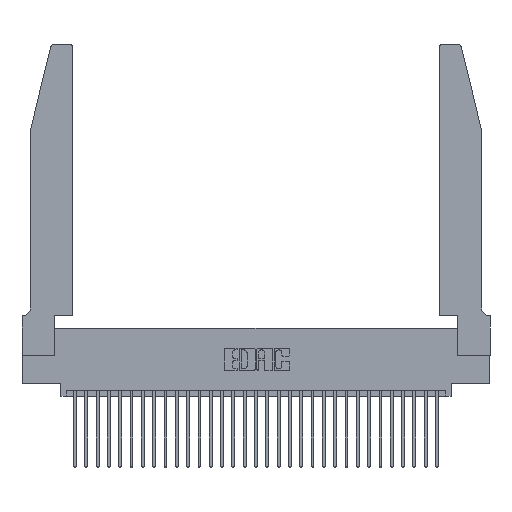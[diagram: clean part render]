
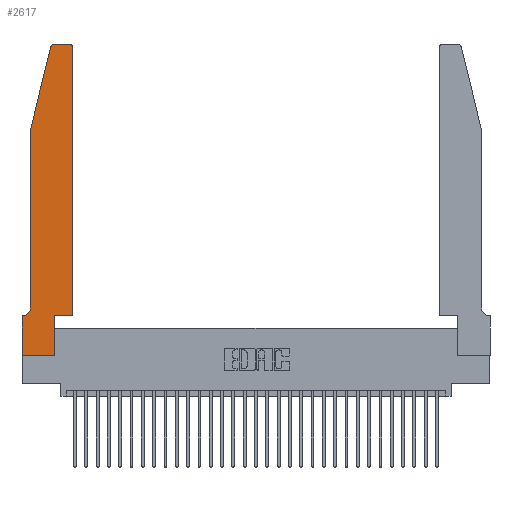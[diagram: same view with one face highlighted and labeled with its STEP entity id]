
A CAD part, top view. The second image highlights one B-rep face of the part: STEP entity #2617.
In plain terms, the highlighted planar face has unit normal (0, 0, 1).
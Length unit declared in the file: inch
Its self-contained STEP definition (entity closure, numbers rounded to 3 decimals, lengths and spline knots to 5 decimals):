
#108 = ORIENTED_EDGE ( 'NONE', *, *, #10033, .T. ) ;
#432 = EDGE_CURVE ( 'NONE', #23651, #25471, #24129, .T. ) ;
#804 = DIRECTION ( 'NONE',  ( 1., 0., 0. ) ) ;
#1020 = CARTESIAN_POINT ( 'NONE',  ( 0., 0., 0.37 ) ) ;
#1551 = DIRECTION ( 'NONE',  ( -1., 0., 0. ) ) ;
#2395 = DIRECTION ( 'NONE',  ( 0., 0., 1. ) ) ;
#2446 = CARTESIAN_POINT ( 'NONE',  ( 0., 0., 0.37 ) ) ;
#2617 = ADVANCED_FACE ( 'NONE', ( #11401 ), #15504, .T. ) ;
#2775 = VECTOR ( 'NONE', #18620, 39.37008 ) ;
#3001 = EDGE_CURVE ( 'NONE', #5700, #26928, #12154, .T. ) ;
#3244 = DIRECTION ( 'NONE',  ( 0., 0., 1. ) ) ;
#3672 = EDGE_LOOP ( 'NONE', ( #5159, #108, #13438, #28857, #13011, #16628, #20167, #29893, #7004, #9780, #23713, #18975 ) ) ;
#4205 = AXIS2_PLACEMENT_3D ( 'NONE', #13001, #25788, #13106 ) ;
#4511 = DIRECTION ( 'NONE',  ( 0., 1., 0. ) ) ;
#4675 = EDGE_CURVE ( 'NONE', #8974, #28708, #5475, .T. ) ;
#4848 = VECTOR ( 'NONE', #4511, 39.37008 ) ;
#5159 = ORIENTED_EDGE ( 'NONE', *, *, #432, .T. ) ;
#5475 = LINE ( 'NONE', #11590, #22478 ) ;
#5673 = CARTESIAN_POINT ( 'NONE',  ( 0.284, 2.75, 0.37 ) ) ;
#5700 = VERTEX_POINT ( 'NONE', #26299 ) ;
#6003 = EDGE_CURVE ( 'NONE', #9294, #23651, #8084, .T. ) ;
#6715 = CARTESIAN_POINT ( 'NONE',  ( 0.0755, 2., 0.37 ) ) ;
#7004 = ORIENTED_EDGE ( 'NONE', *, *, #14526, .T. ) ;
#7499 = VECTOR ( 'NONE', #25709, 39.37008 ) ;
#7746 = VERTEX_POINT ( 'NONE', #14451 ) ;
#7762 = VECTOR ( 'NONE', #28252, 39.37008 ) ;
#8084 = CIRCLE ( 'NONE', #23474, 0.03 ) ;
#8286 = CARTESIAN_POINT ( 'NONE',  ( 0.4205, 2.72, 0.37 ) ) ;
#8386 = CARTESIAN_POINT ( 'NONE',  ( 0.4505, 0.35, 0.37 ) ) ;
#8974 = VERTEX_POINT ( 'NONE', #6715 ) ;
#9065 = CARTESIAN_POINT ( 'NONE',  ( 0.0755, 0.35, 0.37 ) ) ;
#9294 = VERTEX_POINT ( 'NONE', #9440 ) ;
#9440 = CARTESIAN_POINT ( 'NONE',  ( 0.4505, 2.72, 0.37 ) ) ;
#9780 = ORIENTED_EDGE ( 'NONE', *, *, #18970, .T. ) ;
#10033 = EDGE_CURVE ( 'NONE', #25471, #27442, #21724, .T. ) ;
#11401 = FACE_OUTER_BOUND ( 'NONE', #3672, .T. ) ;
#11590 = CARTESIAN_POINT ( 'NONE',  ( 0.0755, 2., 0.37 ) ) ;
#12142 = DIRECTION ( 'NONE',  ( 0., -1., 0. ) ) ;
#12154 = LINE ( 'NONE', #2446, #27236 ) ;
#12492 = DIRECTION ( 'NONE',  ( 0., 0., -1. ) ) ;
#12858 = VERTEX_POINT ( 'NONE', #18215 ) ;
#13001 = CARTESIAN_POINT ( 'NONE',  ( 0., 0.35, 0.37 ) ) ;
#13011 = ORIENTED_EDGE ( 'NONE', *, *, #18200, .T. ) ;
#13106 = DIRECTION ( 'NONE',  ( 1., 0., 0. ) ) ;
#13399 = VECTOR ( 'NONE', #804, 39.37008 ) ;
#13438 = ORIENTED_EDGE ( 'NONE', *, *, #19092, .T. ) ;
#13456 = EDGE_CURVE ( 'NONE', #26928, #12858, #19979, .T. ) ;
#14301 = VECTOR ( 'NONE', #26373, 39.37008 ) ;
#14451 = CARTESIAN_POINT ( 'NONE',  ( 0.2865, 0.35, 0.37 ) ) ;
#14526 = EDGE_CURVE ( 'NONE', #12858, #7746, #31569, .T. ) ;
#14650 = DIRECTION ( 'NONE',  ( -1., 0., 0. ) ) ;
#15427 = CARTESIAN_POINT ( 'NONE',  ( 0.25487, 2.72718, 0.37 ) ) ;
#15504 = PLANE ( 'NONE',  #4205 ) ;
#16032 = VERTEX_POINT ( 'NONE', #28090 ) ;
#16333 = CIRCLE ( 'NONE', #31614, 0.07 ) ;
#16628 = ORIENTED_EDGE ( 'NONE', *, *, #19931, .T. ) ;
#16662 = LINE ( 'NONE', #18415, #7762 ) ;
#17142 = CARTESIAN_POINT ( 'NONE',  ( 0.0055, 0.42, 0.37 ) ) ;
#17158 = CARTESIAN_POINT ( 'NONE',  ( 0.284, 2.72, 0.37 ) ) ;
#17810 = DIRECTION ( 'NONE',  ( 1., 0., 0. ) ) ;
#18200 = EDGE_CURVE ( 'NONE', #28708, #16032, #16333, .T. ) ;
#18215 = CARTESIAN_POINT ( 'NONE',  ( 0.2865, 0., 0.37 ) ) ;
#18336 = LINE ( 'NONE', #8386, #7499 ) ;
#18415 = CARTESIAN_POINT ( 'NONE',  ( 0.4505, 0.35, 0.37 ) ) ;
#18620 = DIRECTION ( 'NONE',  ( -0.239, -0.971, 0. ) ) ;
#18970 = EDGE_CURVE ( 'NONE', #7746, #19333, #16662, .T. ) ;
#18975 = ORIENTED_EDGE ( 'NONE', *, *, #6003, .T. ) ;
#19041 = CARTESIAN_POINT ( 'NONE',  ( 0.2605, 2.75, 0.37 ) ) ;
#19092 = EDGE_CURVE ( 'NONE', #27442, #8974, #22066, .T. ) ;
#19333 = VERTEX_POINT ( 'NONE', #29322 ) ;
#19476 = DIRECTION ( 'NONE',  ( 0., -1., 0. ) ) ;
#19931 = EDGE_CURVE ( 'NONE', #16032, #5700, #31381, .T. ) ;
#19979 = LINE ( 'NONE', #1020, #13399 ) ;
#20167 = ORIENTED_EDGE ( 'NONE', *, *, #3001, .T. ) ;
#20431 = AXIS2_PLACEMENT_3D ( 'NONE', #17158, #2395, #25366 ) ;
#21307 = CARTESIAN_POINT ( 'NONE',  ( 0.0755, 2., 0.37 ) ) ;
#21724 = CIRCLE ( 'NONE', #20431, 0.03 ) ;
#21886 = CARTESIAN_POINT ( 'NONE',  ( 0.2865, 0.35, 0.37 ) ) ;
#22066 = LINE ( 'NONE', #21307, #2775 ) ;
#22478 = VECTOR ( 'NONE', #19476, 39.37008 ) ;
#23474 = AXIS2_PLACEMENT_3D ( 'NONE', #8286, #3244, #17810 ) ;
#23651 = VERTEX_POINT ( 'NONE', #25107 ) ;
#23713 = ORIENTED_EDGE ( 'NONE', *, *, #26663, .T. ) ;
#24129 = LINE ( 'NONE', #19041, #29970 ) ;
#25107 = CARTESIAN_POINT ( 'NONE',  ( 0.4205, 2.75, 0.37 ) ) ;
#25366 = DIRECTION ( 'NONE',  ( 1., 0., 0. ) ) ;
#25471 = VERTEX_POINT ( 'NONE', #5673 ) ;
#25651 = CARTESIAN_POINT ( 'NONE',  ( 0.0755, 0.42, 0.37 ) ) ;
#25709 = DIRECTION ( 'NONE',  ( 0., 1., 0. ) ) ;
#25788 = DIRECTION ( 'NONE',  ( 0., 0., 1. ) ) ;
#26299 = CARTESIAN_POINT ( 'NONE',  ( 0., 0.35, 0.37 ) ) ;
#26373 = DIRECTION ( 'NONE',  ( -1., 0., 0. ) ) ;
#26663 = EDGE_CURVE ( 'NONE', #19333, #9294, #18336, .T. ) ;
#26884 = CARTESIAN_POINT ( 'NONE',  ( 0., 0., 0.37 ) ) ;
#26928 = VERTEX_POINT ( 'NONE', #26884 ) ;
#27236 = VECTOR ( 'NONE', #12142, 39.37008 ) ;
#27442 = VERTEX_POINT ( 'NONE', #15427 ) ;
#28090 = CARTESIAN_POINT ( 'NONE',  ( 0.0055, 0.35, 0.37 ) ) ;
#28252 = DIRECTION ( 'NONE',  ( 1., 0., 0. ) ) ;
#28708 = VERTEX_POINT ( 'NONE', #25651 ) ;
#28857 = ORIENTED_EDGE ( 'NONE', *, *, #4675, .T. ) ;
#29322 = CARTESIAN_POINT ( 'NONE',  ( 0.4505, 0.35, 0.37 ) ) ;
#29893 = ORIENTED_EDGE ( 'NONE', *, *, #13456, .T. ) ;
#29970 = VECTOR ( 'NONE', #1551, 39.37008 ) ;
#31381 = LINE ( 'NONE', #9065, #14301 ) ;
#31569 = LINE ( 'NONE', #21886, #4848 ) ;
#31614 = AXIS2_PLACEMENT_3D ( 'NONE', #17142, #12492, #14650 ) ;
